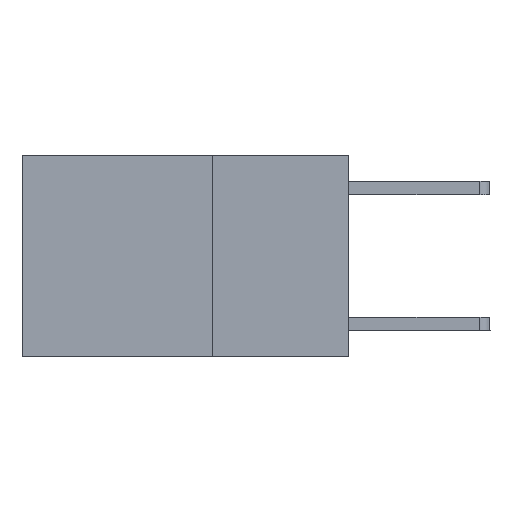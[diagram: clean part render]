
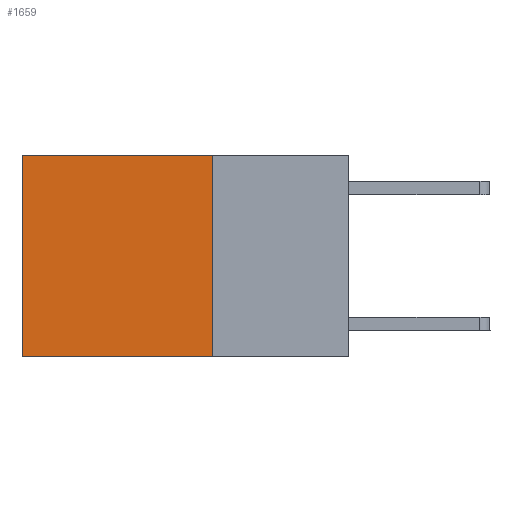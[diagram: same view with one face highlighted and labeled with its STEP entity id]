
A CAD part, left-side view. The second image highlights one B-rep face of the part: STEP entity #1659.
In plain terms, the highlighted planar face has unit normal (-1, 0, 0).
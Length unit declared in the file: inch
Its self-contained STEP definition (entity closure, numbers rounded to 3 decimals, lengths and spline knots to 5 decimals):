
#166 = ORIENTED_EDGE ( 'NONE', *, *, #3301, .F. ) ;
#235 = DIRECTION ( 'NONE',  ( 0., 1., 0. ) ) ;
#696 = CARTESIAN_POINT ( 'NONE',  ( 0.2625, 0.25, -0.37 ) ) ;
#703 = VERTEX_POINT ( 'NONE', #5888 ) ;
#879 = ORIENTED_EDGE ( 'NONE', *, *, #4101, .T. ) ;
#1019 = VECTOR ( 'NONE', #235, 39.37008 ) ;
#1299 = CARTESIAN_POINT ( 'NONE',  ( 0.2625, 0.25, 0. ) ) ;
#1392 = LINE ( 'NONE', #4760, #3560 ) ;
#1522 = DIRECTION ( 'NONE',  ( 0., 1., 0. ) ) ;
#1659 = ADVANCED_FACE ( 'NONE', ( #9520 ), #4446, .F. ) ;
#1684 = VERTEX_POINT ( 'NONE', #9789 ) ;
#1750 = CARTESIAN_POINT ( 'NONE',  ( 0.2625, 0.25, 0. ) ) ;
#2136 = DIRECTION ( 'NONE',  ( 1., 0., 0. ) ) ;
#2825 = VECTOR ( 'NONE', #7750, 39.37008 ) ;
#2877 = LINE ( 'NONE', #7510, #2825 ) ;
#3127 = DIRECTION ( 'NONE',  ( 0., 0., -1. ) ) ;
#3301 = EDGE_CURVE ( 'NONE', #5000, #1684, #2877, .T. ) ;
#3560 = VECTOR ( 'NONE', #9951, 39.37008 ) ;
#4101 = EDGE_CURVE ( 'NONE', #4779, #703, #1392, .T. ) ;
#4112 = LINE ( 'NONE', #696, #6040 ) ;
#4383 = CARTESIAN_POINT ( 'NONE',  ( 0.2625, 0.25, 0. ) ) ;
#4446 = PLANE ( 'NONE',  #6548 ) ;
#4760 = CARTESIAN_POINT ( 'NONE',  ( 0.2625, 0.6, 0. ) ) ;
#4779 = VERTEX_POINT ( 'NONE', #7529 ) ;
#5000 = VERTEX_POINT ( 'NONE', #1750 ) ;
#5719 = ORIENTED_EDGE ( 'NONE', *, *, #8168, .T. ) ;
#5888 = CARTESIAN_POINT ( 'NONE',  ( 0.2625, 0.6, -0.37 ) ) ;
#6040 = VECTOR ( 'NONE', #1522, 39.37008 ) ;
#6548 = AXIS2_PLACEMENT_3D ( 'NONE', #1299, #2136, #3127 ) ;
#6880 = EDGE_LOOP ( 'NONE', ( #879, #7924, #166, #5719 ) ) ;
#7510 = CARTESIAN_POINT ( 'NONE',  ( 0.2625, 0.25, 0. ) ) ;
#7529 = CARTESIAN_POINT ( 'NONE',  ( 0.2625, 0.6, 0. ) ) ;
#7750 = DIRECTION ( 'NONE',  ( 0., 0., -1. ) ) ;
#7924 = ORIENTED_EDGE ( 'NONE', *, *, #9492, .F. ) ;
#8168 = EDGE_CURVE ( 'NONE', #5000, #4779, #9388, .T. ) ;
#9388 = LINE ( 'NONE', #4383, #1019 ) ;
#9492 = EDGE_CURVE ( 'NONE', #1684, #703, #4112, .T. ) ;
#9520 = FACE_OUTER_BOUND ( 'NONE', #6880, .T. ) ;
#9789 = CARTESIAN_POINT ( 'NONE',  ( 0.2625, 0.25, -0.37 ) ) ;
#9951 = DIRECTION ( 'NONE',  ( 0., 0., -1. ) ) ;
